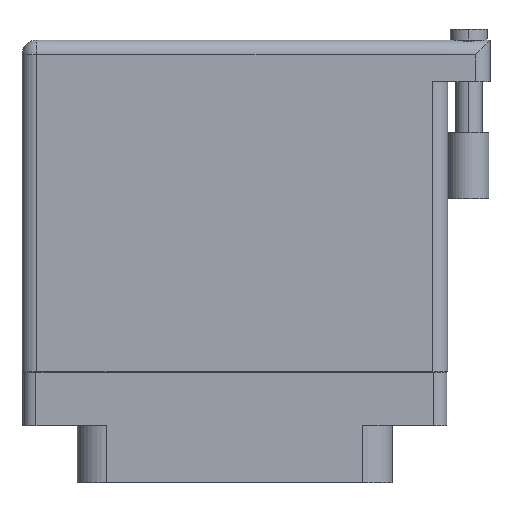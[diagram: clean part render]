
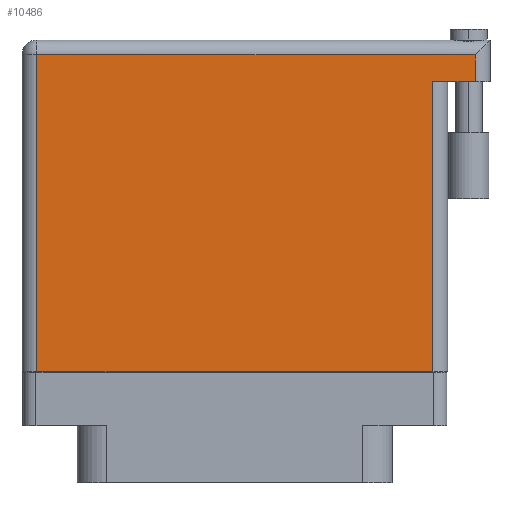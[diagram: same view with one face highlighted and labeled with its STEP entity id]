
A CAD part, front view. The second image highlights one B-rep face of the part: STEP entity #10486.
In plain terms, the highlighted face is planar.
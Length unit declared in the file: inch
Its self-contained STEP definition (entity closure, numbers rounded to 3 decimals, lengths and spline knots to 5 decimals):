
#492 = ORIENTED_EDGE ( 'NONE', *, *, #5377, .T. ) ;
#2805 = PLANE ( 'NONE',  #30729 ) ;
#3570 = CARTESIAN_POINT ( 'NONE',  ( 0.934, 1.269, 0.4495 ) ) ;
#4049 = ORIENTED_EDGE ( 'NONE', *, *, #24707, .F. ) ;
#4060 = LINE ( 'NONE', #33966, #23136 ) ;
#5284 = LINE ( 'NONE', #33674, #35165 ) ;
#5377 = EDGE_CURVE ( 'NONE', #30618, #17645, #4060, .T. ) ;
#6057 = CARTESIAN_POINT ( 'NONE',  ( 0.934, 1.269, 0.4495 ) ) ;
#7076 = CARTESIAN_POINT ( 'NONE',  ( -1.004, 1.396, 0.4495 ) ) ;
#8157 = LINE ( 'NONE', #7076, #32383 ) ;
#8770 = LINE ( 'NONE', #6057, #27411 ) ;
#10486 = ADVANCED_FACE ( 'NONE', ( #23881 ), #2805, .F. ) ;
#11453 = CARTESIAN_POINT ( 'NONE',  ( -0.934, 1.396, 0.4495 ) ) ;
#11784 = DIRECTION ( 'NONE',  ( 0., 1., 0. ) ) ;
#13239 = VERTEX_POINT ( 'NONE', #3570 ) ;
#13455 = CARTESIAN_POINT ( 'NONE',  ( -1.004, 1.466, 0.4495 ) ) ;
#13481 = ORIENTED_EDGE ( 'NONE', *, *, #34616, .T. ) ;
#14079 = EDGE_CURVE ( 'NONE', #25262, #26959, #31832, .T. ) ;
#16960 = CARTESIAN_POINT ( 'NONE',  ( -0.934, -0.1, 0.4495 ) ) ;
#17645 = VERTEX_POINT ( 'NONE', #24089 ) ;
#18624 = CARTESIAN_POINT ( 'NONE',  ( -1.004, -0.1, 0.4495 ) ) ;
#20189 = DIRECTION ( 'NONE',  ( 1., 0., 0. ) ) ;
#20807 = EDGE_LOOP ( 'NONE', ( #24523, #13481, #4049, #492, #33303, #35622 ) ) ;
#21498 = VECTOR ( 'NONE', #22789, 39.37008 ) ;
#21767 = CARTESIAN_POINT ( 'NONE',  ( 0.934, -0.1, 0.4495 ) ) ;
#22789 = DIRECTION ( 'NONE',  ( 0., -1., 0. ) ) ;
#23136 = VECTOR ( 'NONE', #11784, 39.37008 ) ;
#23711 = EDGE_CURVE ( 'NONE', #26959, #28178, #32191, .T. ) ;
#23881 = FACE_OUTER_BOUND ( 'NONE', #20807, .T. ) ;
#24089 = CARTESIAN_POINT ( 'NONE',  ( 1.134, 1.396, 0.4495 ) ) ;
#24523 = ORIENTED_EDGE ( 'NONE', *, *, #23711, .T. ) ;
#24707 = EDGE_CURVE ( 'NONE', #30618, #13239, #5284, .T. ) ;
#25262 = VERTEX_POINT ( 'NONE', #11453 ) ;
#25467 = DIRECTION ( 'NONE',  ( 0., 1., 0. ) ) ;
#26436 = DIRECTION ( 'NONE',  ( -1., 0., 0. ) ) ;
#26959 = VERTEX_POINT ( 'NONE', #28534 ) ;
#27411 = VECTOR ( 'NONE', #25467, 39.37008 ) ;
#27448 = VECTOR ( 'NONE', #20189, 39.37008 ) ;
#27641 = EDGE_CURVE ( 'NONE', #17645, #25262, #8157, .T. ) ;
#28178 = VERTEX_POINT ( 'NONE', #21767 ) ;
#28348 = DIRECTION ( 'NONE',  ( -1., 0., 0. ) ) ;
#28534 = CARTESIAN_POINT ( 'NONE',  ( -0.934, -0.1, 0.4495 ) ) ;
#30156 = DIRECTION ( 'NONE',  ( -1., 0., 0. ) ) ;
#30618 = VERTEX_POINT ( 'NONE', #31496 ) ;
#30729 = AXIS2_PLACEMENT_3D ( 'NONE', #13455, #35625, #30156 ) ;
#31496 = CARTESIAN_POINT ( 'NONE',  ( 1.134, 1.269, 0.4495 ) ) ;
#31832 = LINE ( 'NONE', #16960, #21498 ) ;
#32191 = LINE ( 'NONE', #18624, #27448 ) ;
#32383 = VECTOR ( 'NONE', #26436, 39.37008 ) ;
#33303 = ORIENTED_EDGE ( 'NONE', *, *, #27641, .T. ) ;
#33674 = CARTESIAN_POINT ( 'NONE',  ( 1.204, 1.269, 0.4495 ) ) ;
#33966 = CARTESIAN_POINT ( 'NONE',  ( 1.134, 1.466, 0.4495 ) ) ;
#34616 = EDGE_CURVE ( 'NONE', #28178, #13239, #8770, .T. ) ;
#35165 = VECTOR ( 'NONE', #28348, 39.37008 ) ;
#35622 = ORIENTED_EDGE ( 'NONE', *, *, #14079, .T. ) ;
#35625 = DIRECTION ( 'NONE',  ( 0., 0., -1. ) ) ;
